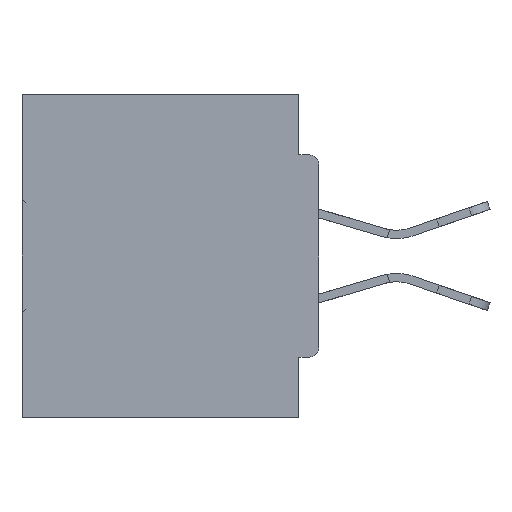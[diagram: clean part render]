
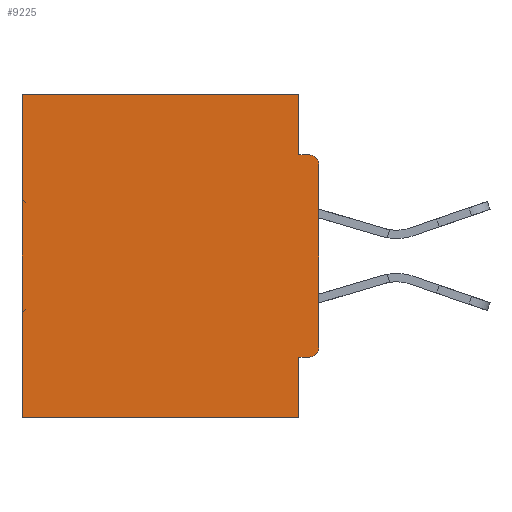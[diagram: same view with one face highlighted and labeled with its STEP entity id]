
A CAD part, left-side view. The second image highlights one B-rep face of the part: STEP entity #9225.
In plain terms, the highlighted planar face has unit normal (-1, 0, 0).
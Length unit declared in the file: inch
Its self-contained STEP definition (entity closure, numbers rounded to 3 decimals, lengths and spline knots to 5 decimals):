
#2524 = VERTEX_POINT ( 'NONE', #43562 ) ;
#2941 = VERTEX_POINT ( 'NONE', #24118 ) ;
#3124 = LINE ( 'NONE', #27407, #24795 ) ;
#3224 = DIRECTION ( 'NONE',  ( 0., 1., 0. ) ) ;
#3463 = DIRECTION ( 'NONE',  ( 0., 1., 0. ) ) ;
#3556 = AXIS2_PLACEMENT_3D ( 'NONE', #44128, #8380, #37438 ) ;
#3693 = VECTOR ( 'NONE', #16190, 39.37008 ) ;
#5069 = ORIENTED_EDGE ( 'NONE', *, *, #16279, .T. ) ;
#5385 = ORIENTED_EDGE ( 'NONE', *, *, #6337, .F. ) ;
#5442 = CARTESIAN_POINT ( 'NONE',  ( 0.298, 0.031, -0.5 ) ) ;
#5792 = AXIS2_PLACEMENT_3D ( 'NONE', #6154, #38072, #31435 ) ;
#6154 = CARTESIAN_POINT ( 'NONE',  ( 0.298, 0.015, -0.1085 ) ) ;
#6337 = EDGE_CURVE ( 'NONE', #8201, #42277, #21506, .T. ) ;
#6638 = VERTEX_POINT ( 'NONE', #9295 ) ;
#8201 = VERTEX_POINT ( 'NONE', #36024 ) ;
#8213 = LINE ( 'NONE', #46025, #25201 ) ;
#8380 = DIRECTION ( 'NONE',  ( 1., 0., 0. ) ) ;
#9156 = EDGE_CURVE ( 'NONE', #6638, #2941, #18865, .T. ) ;
#9225 = ADVANCED_FACE ( 'NONE', ( #28000 ), #29599, .F. ) ;
#9295 = CARTESIAN_POINT ( 'NONE',  ( 0.298, 0.031, -0.0935 ) ) ;
#10156 = ORIENTED_EDGE ( 'NONE', *, *, #40112, .F. ) ;
#11300 = CARTESIAN_POINT ( 'NONE',  ( 0.298, 0.031, -0.4065 ) ) ;
#11473 = CIRCLE ( 'NONE', #26692, 0.015 ) ;
#12206 = CARTESIAN_POINT ( 'NONE',  ( 0.298, 0., -0.1085 ) ) ;
#13239 = ORIENTED_EDGE ( 'NONE', *, *, #15294, .F. ) ;
#13684 = DIRECTION ( 'NONE',  ( -1., 0., 0. ) ) ;
#13845 = LINE ( 'NONE', #15414, #3693 ) ;
#14354 = ORIENTED_EDGE ( 'NONE', *, *, #9156, .F. ) ;
#15294 = EDGE_CURVE ( 'NONE', #20992, #6638, #13845, .T. ) ;
#15414 = CARTESIAN_POINT ( 'NONE',  ( 0.298, 0.031, -0.5 ) ) ;
#15897 = VECTOR ( 'NONE', #17439, 39.37008 ) ;
#16190 = DIRECTION ( 'NONE',  ( 0., 0., -1. ) ) ;
#16279 = EDGE_CURVE ( 'NONE', #20992, #38329, #41465, .T. ) ;
#16701 = CARTESIAN_POINT ( 'NONE',  ( 0.298, 0., -0.4065 ) ) ;
#16740 = DIRECTION ( 'NONE',  ( 0., 0., -1. ) ) ;
#17439 = DIRECTION ( 'NONE',  ( 0., 0., -1. ) ) ;
#17941 = CARTESIAN_POINT ( 'NONE',  ( 0.298, 0., -0.5 ) ) ;
#18027 = ORIENTED_EDGE ( 'NONE', *, *, #25531, .T. ) ;
#18591 = VECTOR ( 'NONE', #42046, 39.37008 ) ;
#18865 = LINE ( 'NONE', #32431, #33055 ) ;
#19394 = VECTOR ( 'NONE', #3224, 39.37008 ) ;
#19955 = CARTESIAN_POINT ( 'NONE',  ( 0.298, 0.031, 0. ) ) ;
#20992 = VERTEX_POINT ( 'NONE', #19955 ) ;
#21506 = LINE ( 'NONE', #16701, #18591 ) ;
#22696 = EDGE_CURVE ( 'NONE', #8201, #2524, #11473, .T. ) ;
#24118 = CARTESIAN_POINT ( 'NONE',  ( 0.298, 0.015, -0.0935 ) ) ;
#24795 = VECTOR ( 'NONE', #16740, 39.37008 ) ;
#24879 = CARTESIAN_POINT ( 'NONE',  ( 0.298, 0., 0. ) ) ;
#25201 = VECTOR ( 'NONE', #28166, 39.37008 ) ;
#25531 = EDGE_CURVE ( 'NONE', #38329, #31506, #3124, .T. ) ;
#25565 = LINE ( 'NONE', #28267, #15897 ) ;
#25590 = CARTESIAN_POINT ( 'NONE',  ( 0.298, 0.015, -0.3915 ) ) ;
#26261 = ORIENTED_EDGE ( 'NONE', *, *, #30857, .F. ) ;
#26692 = AXIS2_PLACEMENT_3D ( 'NONE', #25590, #13684, #46136 ) ;
#26747 = LINE ( 'NONE', #17941, #29019 ) ;
#27407 = CARTESIAN_POINT ( 'NONE',  ( 0.298, 0.46, 0. ) ) ;
#28000 = FACE_OUTER_BOUND ( 'NONE', #33288, .T. ) ;
#28166 = DIRECTION ( 'NONE',  ( 0., 0., -1. ) ) ;
#28267 = CARTESIAN_POINT ( 'NONE',  ( 0.298, 0., 0. ) ) ;
#28792 = CIRCLE ( 'NONE', #5792, 0.015 ) ;
#28914 = ORIENTED_EDGE ( 'NONE', *, *, #36675, .T. ) ;
#29019 = VECTOR ( 'NONE', #3463, 39.37008 ) ;
#29053 = EDGE_CURVE ( 'NONE', #35782, #2524, #25565, .T. ) ;
#29599 = PLANE ( 'NONE',  #3556 ) ;
#30857 = EDGE_CURVE ( 'NONE', #42277, #33272, #8213, .T. ) ;
#31435 = DIRECTION ( 'NONE',  ( 0., 0., -1. ) ) ;
#31506 = VERTEX_POINT ( 'NONE', #40207 ) ;
#32431 = CARTESIAN_POINT ( 'NONE',  ( 0.298, 0., -0.0935 ) ) ;
#32871 = CARTESIAN_POINT ( 'NONE',  ( 0.298, 0.46, 0. ) ) ;
#33055 = VECTOR ( 'NONE', #43188, 39.37008 ) ;
#33272 = VERTEX_POINT ( 'NONE', #5442 ) ;
#33288 = EDGE_LOOP ( 'NONE', ( #28914, #14354, #13239, #5069, #18027, #10156, #26261, #5385, #35176, #46541 ) ) ;
#35176 = ORIENTED_EDGE ( 'NONE', *, *, #22696, .T. ) ;
#35782 = VERTEX_POINT ( 'NONE', #12206 ) ;
#36024 = CARTESIAN_POINT ( 'NONE',  ( 0.298, 0.015, -0.4065 ) ) ;
#36675 = EDGE_CURVE ( 'NONE', #35782, #2941, #28792, .T. ) ;
#37438 = DIRECTION ( 'NONE',  ( 0., 0., -1. ) ) ;
#38072 = DIRECTION ( 'NONE',  ( -1., 0., 0. ) ) ;
#38329 = VERTEX_POINT ( 'NONE', #32871 ) ;
#40112 = EDGE_CURVE ( 'NONE', #33272, #31506, #26747, .T. ) ;
#40207 = CARTESIAN_POINT ( 'NONE',  ( 0.298, 0.46, -0.5 ) ) ;
#41465 = LINE ( 'NONE', #24879, #19394 ) ;
#42046 = DIRECTION ( 'NONE',  ( 0., 1., 0. ) ) ;
#42277 = VERTEX_POINT ( 'NONE', #11300 ) ;
#43188 = DIRECTION ( 'NONE',  ( 0., -1., 0. ) ) ;
#43562 = CARTESIAN_POINT ( 'NONE',  ( 0.298, 0., -0.3915 ) ) ;
#44128 = CARTESIAN_POINT ( 'NONE',  ( 0.298, 0., 0. ) ) ;
#46025 = CARTESIAN_POINT ( 'NONE',  ( 0.298, 0.031, -0.5 ) ) ;
#46136 = DIRECTION ( 'NONE',  ( 0., 0., -1. ) ) ;
#46541 = ORIENTED_EDGE ( 'NONE', *, *, #29053, .F. ) ;
